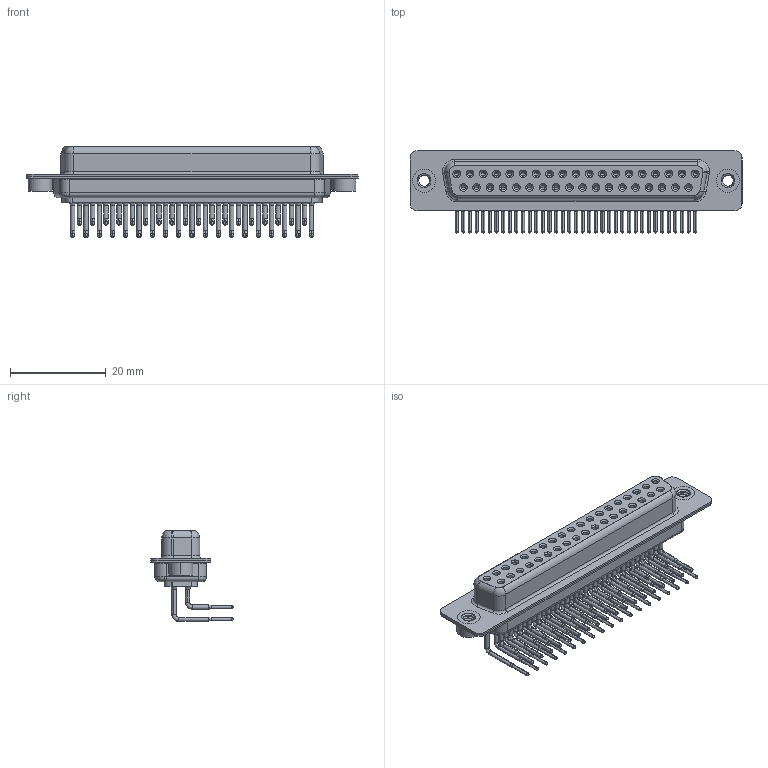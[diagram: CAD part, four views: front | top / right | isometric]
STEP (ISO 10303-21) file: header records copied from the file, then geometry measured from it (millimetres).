
FILE_DESCRIPTION (( 'STEP AP203' ), '1' );
FILE_NAME ('630-M37-240-WT2.STEP', '2018-09-26T04:00:47', ( '' ), ( '' ), 'SwSTEP 2.0', 'SolidWorks 2016', '' );
FILE_SCHEMA (( 'CONFIG_CONTROL_DESIGN' ));
Length unit declared in the file: millimetre
Products named in the file (7): 630M Shell Rear_37 Contacts; 630M Contact Row 1; 630M Contact Row 2; 630M 4-40 Threaded Rivet; 630-M37-240-WT2; 630M Housing_37 Contacts; 630M Shell Front_37 Contacts
Assembly tree (42 placements, depth 2):
  630-M37-240-WT2
    630M Housing_37 Contacts
    630M Shell Front_37 Contacts
    630M Shell Rear_37 Contacts
    630M Contact Row 1  x19
    630M Contact Row 2  x18
    630M 4-40 Threaded Rivet  x2
Bounding box: 69.4 x 17.2 x 18.99 mm (x, y, z)
Volume: 5486.1 mm3; surface area: 13520.9 mm2
Topology: 42 solids, 42 shells, 2240 faces, 5682 edges, 3574 vertices
Faces by surface type: cylinder 988, plane 622, cone 413, bspline 154, torus 63
Entity records: 26734 total; most frequent: CARTESIAN_POINT 5729, DIRECTION 4487, ORIENTED_EDGE 3694, AXIS2_PLACEMENT_3D 1894, EDGE_CURVE 1847, VERTEX_POINT 1176, CIRCLE 1053, EDGE_LOOP 1019
